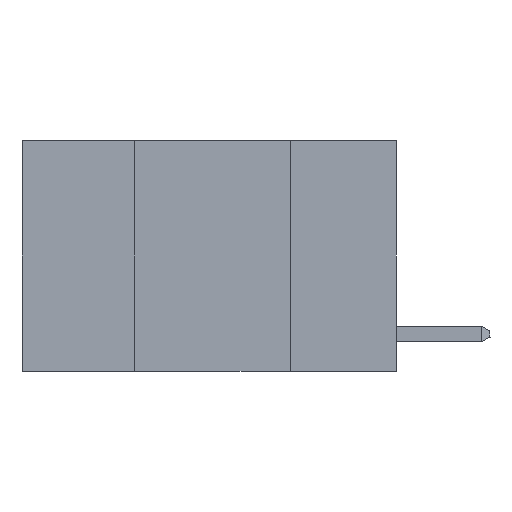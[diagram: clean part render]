
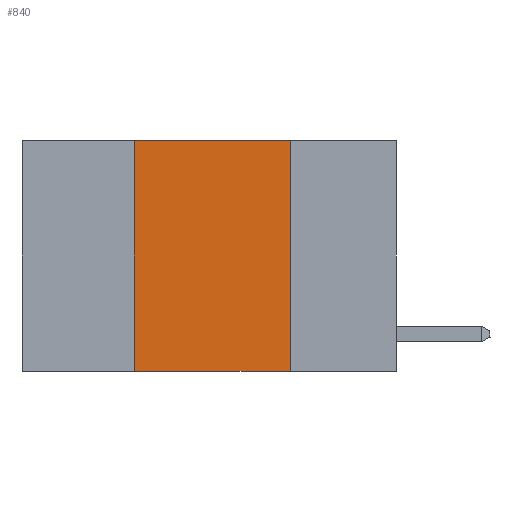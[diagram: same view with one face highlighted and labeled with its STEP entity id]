
A CAD part, left-side view. The second image highlights one B-rep face of the part: STEP entity #840.
In plain terms, the highlighted planar face has unit normal (-1, 0, 0).
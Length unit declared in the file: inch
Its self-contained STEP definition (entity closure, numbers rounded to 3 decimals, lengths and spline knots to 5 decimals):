
#520 = LINE ( 'NONE', #7085, #6429 ) ;
#840 = ADVANCED_FACE ( 'NONE', ( #6457 ), #5945, .F. ) ;
#1071 = CARTESIAN_POINT ( 'NONE',  ( 0., 0.17, 0. ) ) ;
#1113 = DIRECTION ( 'NONE',  ( 0., 0., -1. ) ) ;
#1137 = VERTEX_POINT ( 'NONE', #5549 ) ;
#1301 = EDGE_CURVE ( 'NONE', #2790, #7842, #1314, .T. ) ;
#1314 = LINE ( 'NONE', #3145, #5127 ) ;
#1613 = EDGE_CURVE ( 'NONE', #2790, #1137, #7764, .T. ) ;
#1716 = DIRECTION ( 'NONE',  ( 0., -1., 0. ) ) ;
#1805 = LINE ( 'NONE', #7167, #5502 ) ;
#2384 = EDGE_CURVE ( 'NONE', #7842, #5275, #520, .T. ) ;
#2483 = ORIENTED_EDGE ( 'NONE', *, *, #6382, .F. ) ;
#2490 = DIRECTION ( 'NONE',  ( 0., 0., -1. ) ) ;
#2790 = VERTEX_POINT ( 'NONE', #6999 ) ;
#3089 = DIRECTION ( 'NONE',  ( 0., -1., 0. ) ) ;
#3145 = CARTESIAN_POINT ( 'NONE',  ( 0., 0.42, 0. ) ) ;
#3267 = EDGE_LOOP ( 'NONE', ( #2483, #4607, #8048, #5252 ) ) ;
#3726 = AXIS2_PLACEMENT_3D ( 'NONE', #8458, #6651, #2490 ) ;
#4607 = ORIENTED_EDGE ( 'NONE', *, *, #2384, .F. ) ;
#5127 = VECTOR ( 'NONE', #7967, 39.37008 ) ;
#5252 = ORIENTED_EDGE ( 'NONE', *, *, #1613, .T. ) ;
#5275 = VERTEX_POINT ( 'NONE', #1071 ) ;
#5283 = VECTOR ( 'NONE', #1716, 39.37008 ) ;
#5437 = CARTESIAN_POINT ( 'NONE',  ( 0., 0.42, 0. ) ) ;
#5502 = VECTOR ( 'NONE', #1113, 39.37008 ) ;
#5549 = CARTESIAN_POINT ( 'NONE',  ( 0., 0.17, -0.37 ) ) ;
#5775 = CARTESIAN_POINT ( 'NONE',  ( 0., 0.6, -0.37 ) ) ;
#5945 = PLANE ( 'NONE',  #3726 ) ;
#6382 = EDGE_CURVE ( 'NONE', #5275, #1137, #1805, .T. ) ;
#6429 = VECTOR ( 'NONE', #3089, 39.37008 ) ;
#6457 = FACE_OUTER_BOUND ( 'NONE', #3267, .T. ) ;
#6651 = DIRECTION ( 'NONE',  ( 1., 0., 0. ) ) ;
#6999 = CARTESIAN_POINT ( 'NONE',  ( 0., 0.42, -0.37 ) ) ;
#7085 = CARTESIAN_POINT ( 'NONE',  ( 0., 0.6, 0. ) ) ;
#7167 = CARTESIAN_POINT ( 'NONE',  ( 0., 0.17, 0. ) ) ;
#7764 = LINE ( 'NONE', #5775, #5283 ) ;
#7842 = VERTEX_POINT ( 'NONE', #5437 ) ;
#7967 = DIRECTION ( 'NONE',  ( 0., 0., 1. ) ) ;
#8048 = ORIENTED_EDGE ( 'NONE', *, *, #1301, .F. ) ;
#8458 = CARTESIAN_POINT ( 'NONE',  ( 0., 0.6, 0. ) ) ;
